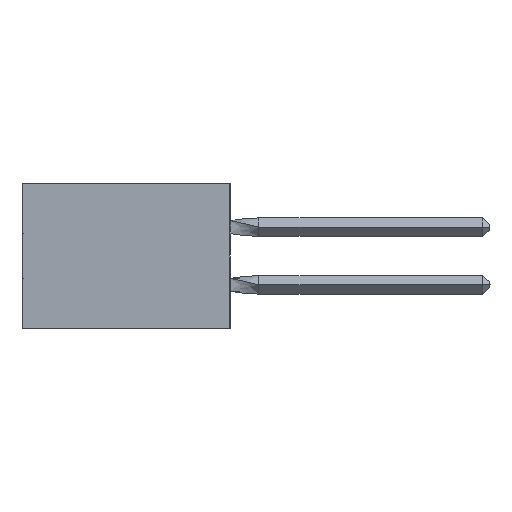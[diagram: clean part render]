
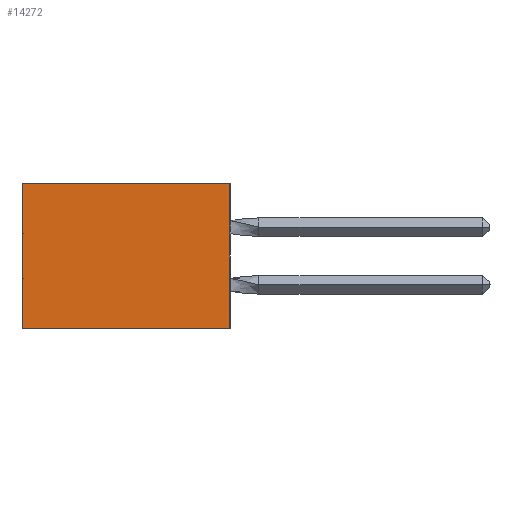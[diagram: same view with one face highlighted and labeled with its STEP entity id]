
A CAD part, left-side view. The second image highlights one B-rep face of the part: STEP entity #14272.
In plain terms, the highlighted planar face has unit normal (-1, 0, 0).
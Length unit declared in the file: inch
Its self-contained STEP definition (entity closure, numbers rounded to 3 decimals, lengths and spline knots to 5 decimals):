
#1096 = VERTEX_POINT ( 'NONE', #44732 ) ;
#1201 = EDGE_LOOP ( 'NONE', ( #45855, #21105, #6754, #28755 ) ) ;
#3999 = CARTESIAN_POINT ( 'NONE',  ( 0.305, 0.72, -0.5 ) ) ;
#4012 = VECTOR ( 'NONE', #32932, 39.37008 ) ;
#4357 = VECTOR ( 'NONE', #15523, 39.37008 ) ;
#5007 = CARTESIAN_POINT ( 'NONE',  ( 0.305, 0., -0.5 ) ) ;
#5214 = PLANE ( 'NONE',  #5808 ) ;
#5808 = AXIS2_PLACEMENT_3D ( 'NONE', #32792, #33506, #16801 ) ;
#6754 = ORIENTED_EDGE ( 'NONE', *, *, #39573, .F. ) ;
#7239 = VERTEX_POINT ( 'NONE', #45189 ) ;
#8532 = CARTESIAN_POINT ( 'NONE',  ( 0.305, 0.72, -0.5 ) ) ;
#10500 = VECTOR ( 'NONE', #41881, 39.37008 ) ;
#13446 = LINE ( 'NONE', #5007, #4012 ) ;
#14272 = ADVANCED_FACE ( 'NONE', ( #48512 ), #5214, .F. ) ;
#15523 = DIRECTION ( 'NONE',  ( 0., 1., 0. ) ) ;
#16801 = DIRECTION ( 'NONE',  ( 0., 0., -1. ) ) ;
#17814 = VECTOR ( 'NONE', #38017, 39.37008 ) ;
#21105 = ORIENTED_EDGE ( 'NONE', *, *, #27596, .F. ) ;
#23864 = CARTESIAN_POINT ( 'NONE',  ( 0.305, 0., -0.5 ) ) ;
#25360 = VERTEX_POINT ( 'NONE', #8532 ) ;
#27596 = EDGE_CURVE ( 'NONE', #34066, #25360, #13446, .T. ) ;
#28755 = ORIENTED_EDGE ( 'NONE', *, *, #35109, .T. ) ;
#30101 = EDGE_CURVE ( 'NONE', #7239, #25360, #32040, .T. ) ;
#32040 = LINE ( 'NONE', #3999, #10500 ) ;
#32792 = CARTESIAN_POINT ( 'NONE',  ( 0.305, 0., -0.5 ) ) ;
#32932 = DIRECTION ( 'NONE',  ( 0., 1., 0. ) ) ;
#33506 = DIRECTION ( 'NONE',  ( 1., 0., 0. ) ) ;
#33680 = CARTESIAN_POINT ( 'NONE',  ( 0.305, 0., -0.5 ) ) ;
#34066 = VERTEX_POINT ( 'NONE', #23864 ) ;
#35109 = EDGE_CURVE ( 'NONE', #1096, #7239, #38603, .T. ) ;
#38017 = DIRECTION ( 'NONE',  ( 0., 0., -1. ) ) ;
#38603 = LINE ( 'NONE', #43881, #4357 ) ;
#39573 = EDGE_CURVE ( 'NONE', #1096, #34066, #51394, .T. ) ;
#41881 = DIRECTION ( 'NONE',  ( 0., 0., -1. ) ) ;
#43881 = CARTESIAN_POINT ( 'NONE',  ( 0.305, 0., 0. ) ) ;
#44732 = CARTESIAN_POINT ( 'NONE',  ( 0.305, 0., 0. ) ) ;
#45189 = CARTESIAN_POINT ( 'NONE',  ( 0.305, 0.72, 0. ) ) ;
#45855 = ORIENTED_EDGE ( 'NONE', *, *, #30101, .T. ) ;
#48512 = FACE_OUTER_BOUND ( 'NONE', #1201, .T. ) ;
#51394 = LINE ( 'NONE', #33680, #17814 ) ;
